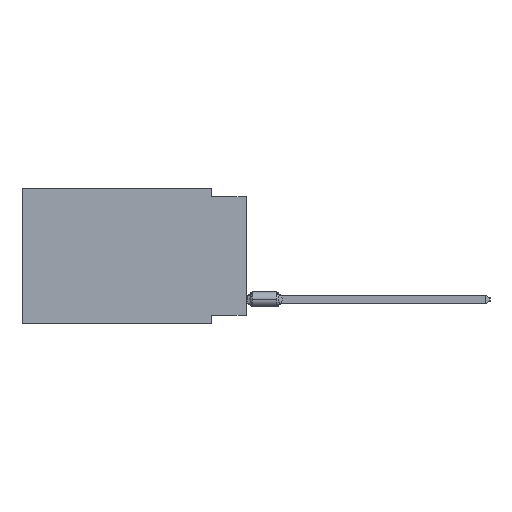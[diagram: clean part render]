
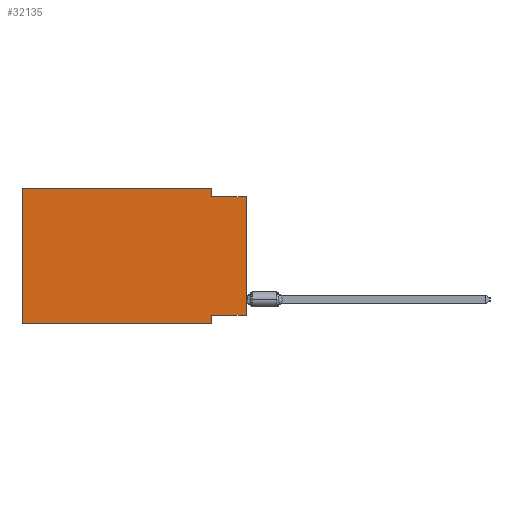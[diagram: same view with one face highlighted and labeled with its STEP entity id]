
A CAD part, left-side view. The second image highlights one B-rep face of the part: STEP entity #32135.
In plain terms, the highlighted planar face has unit normal (-1, 0, 0).
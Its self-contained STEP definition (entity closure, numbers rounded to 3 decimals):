
#252 = CARTESIAN_POINT ( 'NONE',  ( 0., 16.383, 0. ) ) ;
#347 = EDGE_CURVE ( 'NONE', #54596, #34758, #17054, .T. ) ;
#699 = VERTEX_POINT ( 'NONE', #42002 ) ;
#1097 = EDGE_CURVE ( 'NONE', #2648, #30946, #13027, .T. ) ;
#2110 = ORIENTED_EDGE ( 'NONE', *, *, #347, .F. ) ;
#2449 = EDGE_LOOP ( 'NONE', ( #19620, #27842, #57712, #60535, #3415, #53817, #41381, #2110 ) ) ;
#2571 = DIRECTION ( 'NONE',  ( 0., -1., 0. ) ) ;
#2648 = VERTEX_POINT ( 'NONE', #41700 ) ;
#3415 = ORIENTED_EDGE ( 'NONE', *, *, #13534, .F. ) ;
#3823 = DIRECTION ( 'NONE',  ( 0., 0., -1. ) ) ;
#5261 = DIRECTION ( 'NONE',  ( 0., 0., 1. ) ) ;
#5323 = EDGE_CURVE ( 'NONE', #46176, #31667, #22053, .T. ) ;
#5607 = EDGE_CURVE ( 'NONE', #34758, #699, #41839, .T. ) ;
#8563 = DIRECTION ( 'NONE',  ( 0., 0., -1. ) ) ;
#10530 = CARTESIAN_POINT ( 'NONE',  ( 0., 0., -0.635 ) ) ;
#13027 = LINE ( 'NONE', #22457, #60817 ) ;
#13534 = EDGE_CURVE ( 'NONE', #38821, #46176, #34768, .T. ) ;
#15656 = AXIS2_PLACEMENT_3D ( 'NONE', #17999, #18620, #8563 ) ;
#17054 = LINE ( 'NONE', #39986, #52688 ) ;
#17970 = CARTESIAN_POINT ( 'NONE',  ( 0., 2.54, -9.906 ) ) ;
#17999 = CARTESIAN_POINT ( 'NONE',  ( 0., 16.383, 0. ) ) ;
#18309 = PLANE ( 'NONE',  #15656 ) ;
#18620 = DIRECTION ( 'NONE',  ( 1., 0., 0. ) ) ;
#18966 = CARTESIAN_POINT ( 'NONE',  ( 0., 16.383, 0. ) ) ;
#19620 = ORIENTED_EDGE ( 'NONE', *, *, #46583, .T. ) ;
#20035 = DIRECTION ( 'NONE',  ( 0., 0., 1. ) ) ;
#22053 = LINE ( 'NONE', #32109, #48112 ) ;
#22457 = CARTESIAN_POINT ( 'NONE',  ( 0., 0., -0.635 ) ) ;
#24750 = CARTESIAN_POINT ( 'NONE',  ( 0., 0., 0. ) ) ;
#25944 = EDGE_CURVE ( 'NONE', #38821, #699, #32592, .T. ) ;
#27842 = ORIENTED_EDGE ( 'NONE', *, *, #1097, .F. ) ;
#27937 = DIRECTION ( 'NONE',  ( 0., 0., -1. ) ) ;
#30075 = VECTOR ( 'NONE', #3823, 1000. ) ;
#30946 = VERTEX_POINT ( 'NONE', #10530 ) ;
#31667 = VERTEX_POINT ( 'NONE', #56701 ) ;
#31752 = CARTESIAN_POINT ( 'NONE',  ( 0., 2.54, -9.271 ) ) ;
#32109 = CARTESIAN_POINT ( 'NONE',  ( 0., 16.383, 0. ) ) ;
#32135 = ADVANCED_FACE ( 'NONE', ( #46882 ), #18309, .F. ) ;
#32592 = LINE ( 'NONE', #41697, #52335 ) ;
#34695 = CARTESIAN_POINT ( 'NONE',  ( 0., 0., -9.271 ) ) ;
#34758 = VERTEX_POINT ( 'NONE', #31752 ) ;
#34768 = LINE ( 'NONE', #252, #38738 ) ;
#36220 = DIRECTION ( 'NONE',  ( 0., 1., 0. ) ) ;
#37222 = DIRECTION ( 'NONE',  ( 0., -1., 0. ) ) ;
#38738 = VECTOR ( 'NONE', #5261, 1000. ) ;
#38821 = VERTEX_POINT ( 'NONE', #44879 ) ;
#39986 = CARTESIAN_POINT ( 'NONE',  ( 0., 0., -9.271 ) ) ;
#41381 = ORIENTED_EDGE ( 'NONE', *, *, #5607, .F. ) ;
#41697 = CARTESIAN_POINT ( 'NONE',  ( 0., 16.383, -9.906 ) ) ;
#41700 = CARTESIAN_POINT ( 'NONE',  ( 0., 2.54, -0.635 ) ) ;
#41839 = LINE ( 'NONE', #17970, #30075 ) ;
#42002 = CARTESIAN_POINT ( 'NONE',  ( 0., 2.54, -9.906 ) ) ;
#42073 = CARTESIAN_POINT ( 'NONE',  ( 0., 2.54, 0. ) ) ;
#44879 = CARTESIAN_POINT ( 'NONE',  ( 0., 16.383, -9.906 ) ) ;
#46086 = DIRECTION ( 'NONE',  ( 0., -1., 0. ) ) ;
#46176 = VERTEX_POINT ( 'NONE', #18966 ) ;
#46419 = VECTOR ( 'NONE', #20035, 1000. ) ;
#46583 = EDGE_CURVE ( 'NONE', #54596, #30946, #52696, .T. ) ;
#46882 = FACE_OUTER_BOUND ( 'NONE', #2449, .T. ) ;
#48112 = VECTOR ( 'NONE', #2571, 1000. ) ;
#50253 = VECTOR ( 'NONE', #27937, 1000. ) ;
#52335 = VECTOR ( 'NONE', #46086, 1000. ) ;
#52688 = VECTOR ( 'NONE', #36220, 1000. ) ;
#52696 = LINE ( 'NONE', #24750, #46419 ) ;
#53817 = ORIENTED_EDGE ( 'NONE', *, *, #25944, .T. ) ;
#54596 = VERTEX_POINT ( 'NONE', #34695 ) ;
#55091 = EDGE_CURVE ( 'NONE', #31667, #2648, #56813, .T. ) ;
#56701 = CARTESIAN_POINT ( 'NONE',  ( 0., 2.54, 0. ) ) ;
#56813 = LINE ( 'NONE', #42073, #50253 ) ;
#57712 = ORIENTED_EDGE ( 'NONE', *, *, #55091, .F. ) ;
#60535 = ORIENTED_EDGE ( 'NONE', *, *, #5323, .F. ) ;
#60817 = VECTOR ( 'NONE', #37222, 1000. ) ;
